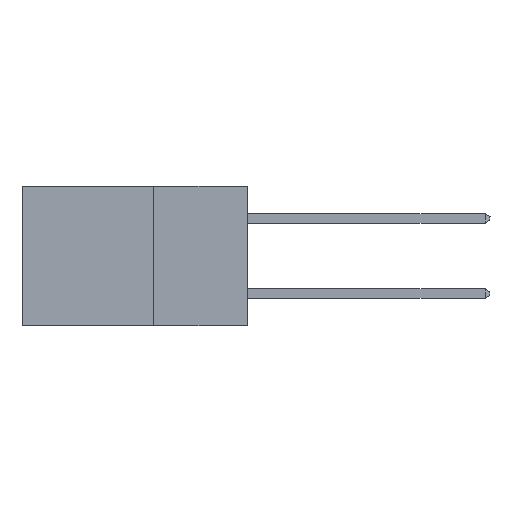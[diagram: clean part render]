
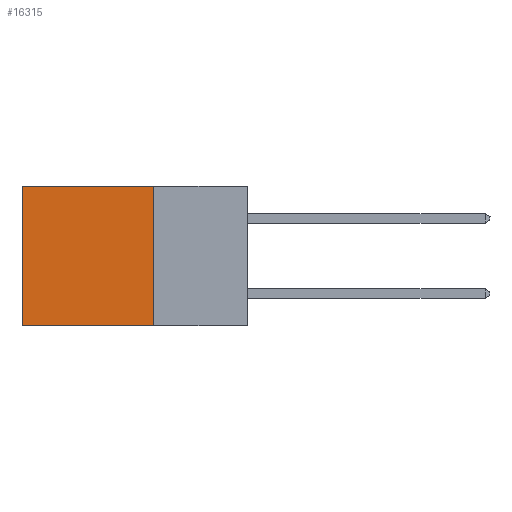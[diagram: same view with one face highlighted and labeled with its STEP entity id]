
A CAD part, left-side view. The second image highlights one B-rep face of the part: STEP entity #16315.
In plain terms, the highlighted planar face has unit normal (-1, 0, 0).
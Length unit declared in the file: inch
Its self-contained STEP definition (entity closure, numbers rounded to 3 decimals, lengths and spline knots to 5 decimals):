
#780 = CARTESIAN_POINT ( 'NONE',  ( 0.298, 0.6, 0. ) ) ;
#1245 = CARTESIAN_POINT ( 'NONE',  ( 0.298, 0.25, 0. ) ) ;
#1300 = DIRECTION ( 'NONE',  ( 0., 0., -1. ) ) ;
#1602 = DIRECTION ( 'NONE',  ( 0., 1., 0. ) ) ;
#1619 = ORIENTED_EDGE ( 'NONE', *, *, #9186, .T. ) ;
#2402 = LINE ( 'NONE', #9508, #16046 ) ;
#2848 = ORIENTED_EDGE ( 'NONE', *, *, #16694, .T. ) ;
#3380 = DIRECTION ( 'NONE',  ( 0., 0., -1. ) ) ;
#3480 = EDGE_CURVE ( 'NONE', #12062, #7922, #2402, .T. ) ;
#4010 = CARTESIAN_POINT ( 'NONE',  ( 0.298, 0.25, 0. ) ) ;
#4765 = VERTEX_POINT ( 'NONE', #4010 ) ;
#5000 = EDGE_LOOP ( 'NONE', ( #1619, #14977, #13223, #2848 ) ) ;
#5981 = LINE ( 'NONE', #11023, #9851 ) ;
#7438 = LINE ( 'NONE', #8588, #14074 ) ;
#7612 = CARTESIAN_POINT ( 'NONE',  ( 0.298, 0.25, 0. ) ) ;
#7695 = VERTEX_POINT ( 'NONE', #780 ) ;
#7922 = VERTEX_POINT ( 'NONE', #8270 ) ;
#8134 = LINE ( 'NONE', #1245, #9782 ) ;
#8270 = CARTESIAN_POINT ( 'NONE',  ( 0.298, 0.6, -0.37 ) ) ;
#8588 = CARTESIAN_POINT ( 'NONE',  ( 0.298, 0.6, 0. ) ) ;
#8999 = DIRECTION ( 'NONE',  ( 1., 0., 0. ) ) ;
#9186 = EDGE_CURVE ( 'NONE', #7695, #7922, #7438, .T. ) ;
#9508 = CARTESIAN_POINT ( 'NONE',  ( 0.298, 0.25, -0.37 ) ) ;
#9606 = FACE_OUTER_BOUND ( 'NONE', #5000, .T. ) ;
#9646 = CARTESIAN_POINT ( 'NONE',  ( 0.298, 0.25, -0.37 ) ) ;
#9782 = VECTOR ( 'NONE', #12897, 39.37008 ) ;
#9851 = VECTOR ( 'NONE', #12488, 39.37008 ) ;
#11023 = CARTESIAN_POINT ( 'NONE',  ( 0.298, 0.25, 0. ) ) ;
#12062 = VERTEX_POINT ( 'NONE', #9646 ) ;
#12488 = DIRECTION ( 'NONE',  ( 0., 0., -1. ) ) ;
#12897 = DIRECTION ( 'NONE',  ( 0., 1., 0. ) ) ;
#13223 = ORIENTED_EDGE ( 'NONE', *, *, #14736, .F. ) ;
#14074 = VECTOR ( 'NONE', #3380, 39.37008 ) ;
#14352 = PLANE ( 'NONE',  #16696 ) ;
#14736 = EDGE_CURVE ( 'NONE', #4765, #12062, #5981, .T. ) ;
#14977 = ORIENTED_EDGE ( 'NONE', *, *, #3480, .F. ) ;
#16046 = VECTOR ( 'NONE', #1602, 39.37008 ) ;
#16315 = ADVANCED_FACE ( 'NONE', ( #9606 ), #14352, .F. ) ;
#16694 = EDGE_CURVE ( 'NONE', #4765, #7695, #8134, .T. ) ;
#16696 = AXIS2_PLACEMENT_3D ( 'NONE', #7612, #8999, #1300 ) ;
